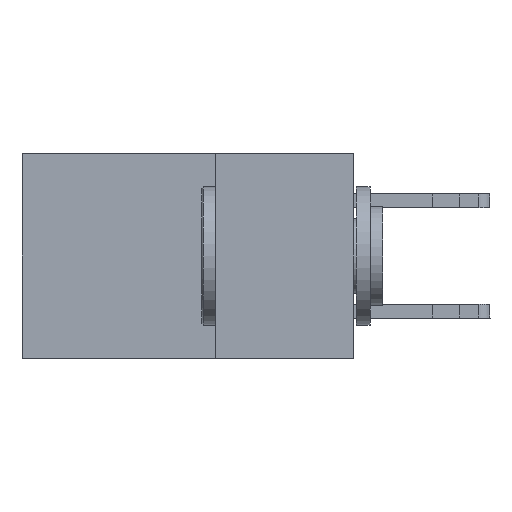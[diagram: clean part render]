
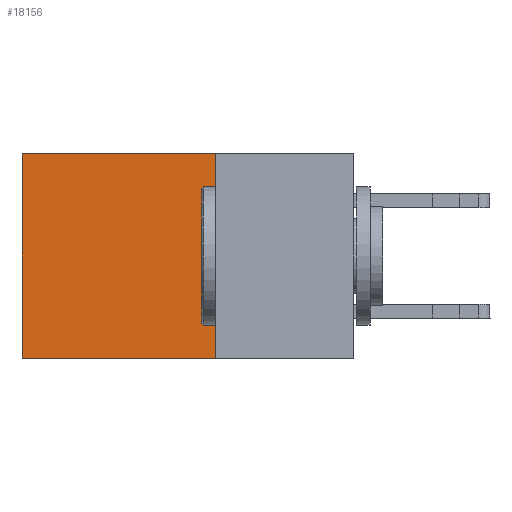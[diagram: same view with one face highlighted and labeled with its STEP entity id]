
A CAD part, left-side view. The second image highlights one B-rep face of the part: STEP entity #18156.
In plain terms, the highlighted planar face has unit normal (-1, 0, 0).
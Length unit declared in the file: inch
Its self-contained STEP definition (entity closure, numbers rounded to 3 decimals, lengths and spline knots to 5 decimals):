
#684 = CARTESIAN_POINT ( 'NONE',  ( 0.2875, 0.25, 0. ) ) ;
#810 = CARTESIAN_POINT ( 'NONE',  ( 0.2875, 0.6, 0. ) ) ;
#1030 = CARTESIAN_POINT ( 'NONE',  ( 0.2875, 0.25, -0.37 ) ) ;
#2151 = FACE_OUTER_BOUND ( 'NONE', #12841, .T. ) ;
#2879 = CARTESIAN_POINT ( 'NONE',  ( 0.2875, 0.6, -0.37 ) ) ;
#3669 = LINE ( 'NONE', #15998, #11311 ) ;
#4150 = DIRECTION ( 'NONE',  ( 0., 1., 0. ) ) ;
#4486 = AXIS2_PLACEMENT_3D ( 'NONE', #15696, #6405, #17193 ) ;
#5331 = CARTESIAN_POINT ( 'NONE',  ( 0.2875, 0.25, 0. ) ) ;
#5471 = VERTEX_POINT ( 'NONE', #12052 ) ;
#5473 = VERTEX_POINT ( 'NONE', #2879 ) ;
#5615 = LINE ( 'NONE', #19094, #17416 ) ;
#6405 = DIRECTION ( 'NONE',  ( 1., 0., 0. ) ) ;
#7107 = ORIENTED_EDGE ( 'NONE', *, *, #8609, .F. ) ;
#7569 = VERTEX_POINT ( 'NONE', #810 ) ;
#8067 = ORIENTED_EDGE ( 'NONE', *, *, #13964, .T. ) ;
#8609 = EDGE_CURVE ( 'NONE', #18977, #5471, #3669, .T. ) ;
#9883 = DIRECTION ( 'NONE',  ( 0., 0., -1. ) ) ;
#10438 = EDGE_CURVE ( 'NONE', #5471, #5473, #12258, .T. ) ;
#11311 = VECTOR ( 'NONE', #14488, 39.37008 ) ;
#12052 = CARTESIAN_POINT ( 'NONE',  ( 0.2875, 0.25, -0.37 ) ) ;
#12258 = LINE ( 'NONE', #1030, #19903 ) ;
#12715 = ORIENTED_EDGE ( 'NONE', *, *, #10438, .F. ) ;
#12841 = EDGE_LOOP ( 'NONE', ( #8067, #12715, #7107, #15416 ) ) ;
#12860 = LINE ( 'NONE', #684, #16445 ) ;
#13044 = DIRECTION ( 'NONE',  ( 0., 1., 0. ) ) ;
#13375 = EDGE_CURVE ( 'NONE', #18977, #7569, #12860, .T. ) ;
#13964 = EDGE_CURVE ( 'NONE', #7569, #5473, #5615, .T. ) ;
#14488 = DIRECTION ( 'NONE',  ( 0., 0., -1. ) ) ;
#15416 = ORIENTED_EDGE ( 'NONE', *, *, #13375, .T. ) ;
#15648 = PLANE ( 'NONE',  #4486 ) ;
#15696 = CARTESIAN_POINT ( 'NONE',  ( 0.2875, 0.25, 0. ) ) ;
#15998 = CARTESIAN_POINT ( 'NONE',  ( 0.2875, 0.25, 0. ) ) ;
#16445 = VECTOR ( 'NONE', #13044, 39.37008 ) ;
#17193 = DIRECTION ( 'NONE',  ( 0., 0., -1. ) ) ;
#17416 = VECTOR ( 'NONE', #9883, 39.37008 ) ;
#18156 = ADVANCED_FACE ( 'NONE', ( #2151 ), #15648, .F. ) ;
#18977 = VERTEX_POINT ( 'NONE', #5331 ) ;
#19094 = CARTESIAN_POINT ( 'NONE',  ( 0.2875, 0.6, 0. ) ) ;
#19903 = VECTOR ( 'NONE', #4150, 39.37008 ) ;
